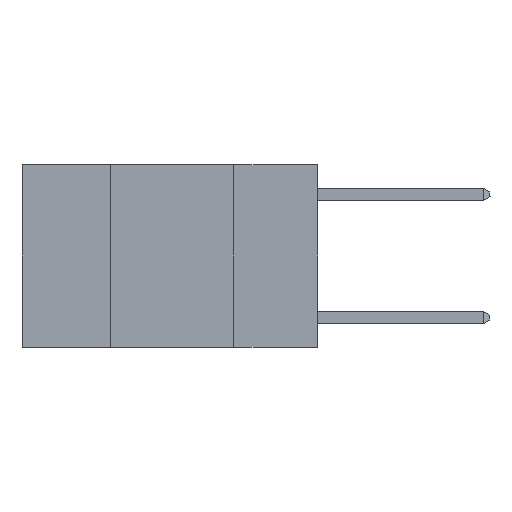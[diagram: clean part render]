
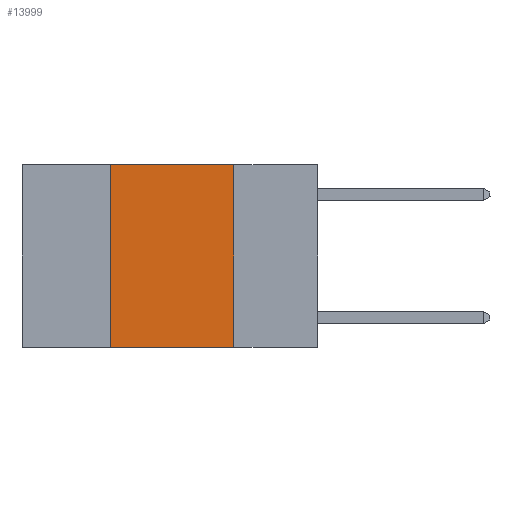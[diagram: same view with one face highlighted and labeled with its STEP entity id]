
A CAD part, left-side view. The second image highlights one B-rep face of the part: STEP entity #13999.
In plain terms, the highlighted planar face has unit normal (-1, 0, 0).
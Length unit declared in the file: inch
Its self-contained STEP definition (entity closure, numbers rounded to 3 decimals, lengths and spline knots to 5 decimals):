
#54 = ORIENTED_EDGE ( 'NONE', *, *, #5010, .F. ) ;
#542 = ORIENTED_EDGE ( 'NONE', *, *, #10276, .F. ) ;
#780 = AXIS2_PLACEMENT_3D ( 'NONE', #896, #8481, #1997 ) ;
#788 = ORIENTED_EDGE ( 'NONE', *, *, #10656, .F. ) ;
#877 = CARTESIAN_POINT ( 'NONE',  ( 0., 0.6, -0.37 ) ) ;
#891 = CARTESIAN_POINT ( 'NONE',  ( 0., 0.42, -0.37 ) ) ;
#896 = CARTESIAN_POINT ( 'NONE',  ( 0., 0.6, 0. ) ) ;
#923 = ORIENTED_EDGE ( 'NONE', *, *, #7252, .T. ) ;
#1596 = EDGE_LOOP ( 'NONE', ( #54, #788, #542, #923 ) ) ;
#1746 = DIRECTION ( 'NONE',  ( 0., 0., 1. ) ) ;
#1972 = VERTEX_POINT ( 'NONE', #10601 ) ;
#1997 = DIRECTION ( 'NONE',  ( 0., 0., -1. ) ) ;
#2435 = VECTOR ( 'NONE', #4513, 39.37008 ) ;
#2562 = CARTESIAN_POINT ( 'NONE',  ( 0., 0.42, 0. ) ) ;
#3119 = VECTOR ( 'NONE', #3722, 39.37008 ) ;
#3454 = CARTESIAN_POINT ( 'NONE',  ( 0., 0.6, 0. ) ) ;
#3460 = LINE ( 'NONE', #13569, #3119 ) ;
#3722 = DIRECTION ( 'NONE',  ( 0., 0., -1. ) ) ;
#4017 = VERTEX_POINT ( 'NONE', #2562 ) ;
#4281 = VECTOR ( 'NONE', #1746, 39.37008 ) ;
#4513 = DIRECTION ( 'NONE',  ( 0., -1., 0. ) ) ;
#5010 = EDGE_CURVE ( 'NONE', #6456, #1972, #3460, .T. ) ;
#6456 = VERTEX_POINT ( 'NONE', #12817 ) ;
#7162 = LINE ( 'NONE', #13627, #4281 ) ;
#7252 = EDGE_CURVE ( 'NONE', #8614, #1972, #7261, .T. ) ;
#7261 = LINE ( 'NONE', #877, #12579 ) ;
#7353 = DIRECTION ( 'NONE',  ( 0., -1., 0. ) ) ;
#8481 = DIRECTION ( 'NONE',  ( 1., 0., 0. ) ) ;
#8614 = VERTEX_POINT ( 'NONE', #891 ) ;
#10276 = EDGE_CURVE ( 'NONE', #8614, #4017, #7162, .T. ) ;
#10408 = FACE_OUTER_BOUND ( 'NONE', #1596, .T. ) ;
#10601 = CARTESIAN_POINT ( 'NONE',  ( 0., 0.17, -0.37 ) ) ;
#10656 = EDGE_CURVE ( 'NONE', #4017, #6456, #11130, .T. ) ;
#11130 = LINE ( 'NONE', #3454, #2435 ) ;
#12579 = VECTOR ( 'NONE', #7353, 39.37008 ) ;
#12817 = CARTESIAN_POINT ( 'NONE',  ( 0., 0.17, 0. ) ) ;
#12871 = PLANE ( 'NONE',  #780 ) ;
#13569 = CARTESIAN_POINT ( 'NONE',  ( 0., 0.17, 0. ) ) ;
#13627 = CARTESIAN_POINT ( 'NONE',  ( 0., 0.42, 0. ) ) ;
#13999 = ADVANCED_FACE ( 'NONE', ( #10408 ), #12871, .F. ) ;
